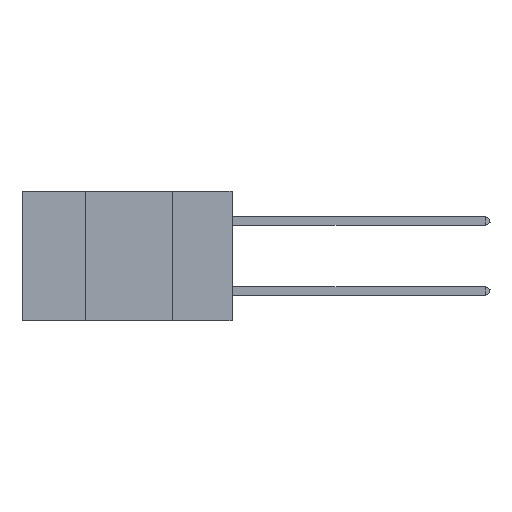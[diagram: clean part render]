
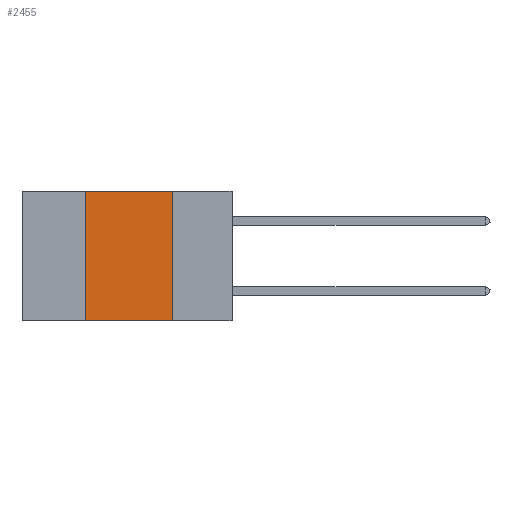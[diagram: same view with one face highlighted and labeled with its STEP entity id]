
A CAD part, left-side view. The second image highlights one B-rep face of the part: STEP entity #2455.
In plain terms, the highlighted planar face has unit normal (-1, 0, 0).
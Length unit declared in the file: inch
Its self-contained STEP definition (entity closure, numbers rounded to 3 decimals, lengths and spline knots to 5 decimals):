
#178 = EDGE_CURVE ( 'NONE', #2836, #7764, #16419, .T. ) ;
#182 = VERTEX_POINT ( 'NONE', #14640 ) ;
#873 = EDGE_CURVE ( 'NONE', #7764, #4798, #7429, .T. ) ;
#1305 = DIRECTION ( 'NONE',  ( 0., 0., -1. ) ) ;
#2210 = LINE ( 'NONE', #20532, #19552 ) ;
#2455 = ADVANCED_FACE ( 'NONE', ( #2963 ), #6495, .F. ) ;
#2549 = EDGE_CURVE ( 'NONE', #4798, #182, #5942, .T. ) ;
#2819 = VECTOR ( 'NONE', #21503, 39.37008 ) ;
#2836 = VERTEX_POINT ( 'NONE', #16351 ) ;
#2963 = FACE_OUTER_BOUND ( 'NONE', #9029, .T. ) ;
#3316 = DIRECTION ( 'NONE',  ( 0., 0., -1. ) ) ;
#4798 = VERTEX_POINT ( 'NONE', #8448 ) ;
#5882 = CARTESIAN_POINT ( 'NONE',  ( 0., 0.42, 0. ) ) ;
#5942 = LINE ( 'NONE', #13718, #15173 ) ;
#6317 = ORIENTED_EDGE ( 'NONE', *, *, #21520, .T. ) ;
#6495 = PLANE ( 'NONE',  #11663 ) ;
#7124 = ORIENTED_EDGE ( 'NONE', *, *, #873, .F. ) ;
#7429 = LINE ( 'NONE', #19787, #2819 ) ;
#7764 = VERTEX_POINT ( 'NONE', #5882 ) ;
#8444 = DIRECTION ( 'NONE',  ( 0., -1., 0. ) ) ;
#8448 = CARTESIAN_POINT ( 'NONE',  ( 0., 0.17, 0. ) ) ;
#9029 = EDGE_LOOP ( 'NONE', ( #18767, #7124, #17969, #6317 ) ) ;
#11149 = CARTESIAN_POINT ( 'NONE',  ( 0., 0.42, 0. ) ) ;
#11663 = AXIS2_PLACEMENT_3D ( 'NONE', #22019, #11754, #1305 ) ;
#11754 = DIRECTION ( 'NONE',  ( 1., 0., 0. ) ) ;
#13718 = CARTESIAN_POINT ( 'NONE',  ( 0., 0.17, 0. ) ) ;
#14640 = CARTESIAN_POINT ( 'NONE',  ( 0., 0.17, -0.37 ) ) ;
#15173 = VECTOR ( 'NONE', #3316, 39.37008 ) ;
#16351 = CARTESIAN_POINT ( 'NONE',  ( 0., 0.42, -0.37 ) ) ;
#16419 = LINE ( 'NONE', #11149, #16970 ) ;
#16970 = VECTOR ( 'NONE', #19745, 39.37008 ) ;
#17969 = ORIENTED_EDGE ( 'NONE', *, *, #178, .F. ) ;
#18767 = ORIENTED_EDGE ( 'NONE', *, *, #2549, .F. ) ;
#19552 = VECTOR ( 'NONE', #8444, 39.37008 ) ;
#19745 = DIRECTION ( 'NONE',  ( 0., 0., 1. ) ) ;
#19787 = CARTESIAN_POINT ( 'NONE',  ( 0., 0.6, 0. ) ) ;
#20532 = CARTESIAN_POINT ( 'NONE',  ( 0., 0.6, -0.37 ) ) ;
#21503 = DIRECTION ( 'NONE',  ( 0., -1., 0. ) ) ;
#21520 = EDGE_CURVE ( 'NONE', #2836, #182, #2210, .T. ) ;
#22019 = CARTESIAN_POINT ( 'NONE',  ( 0., 0.6, 0. ) ) ;
